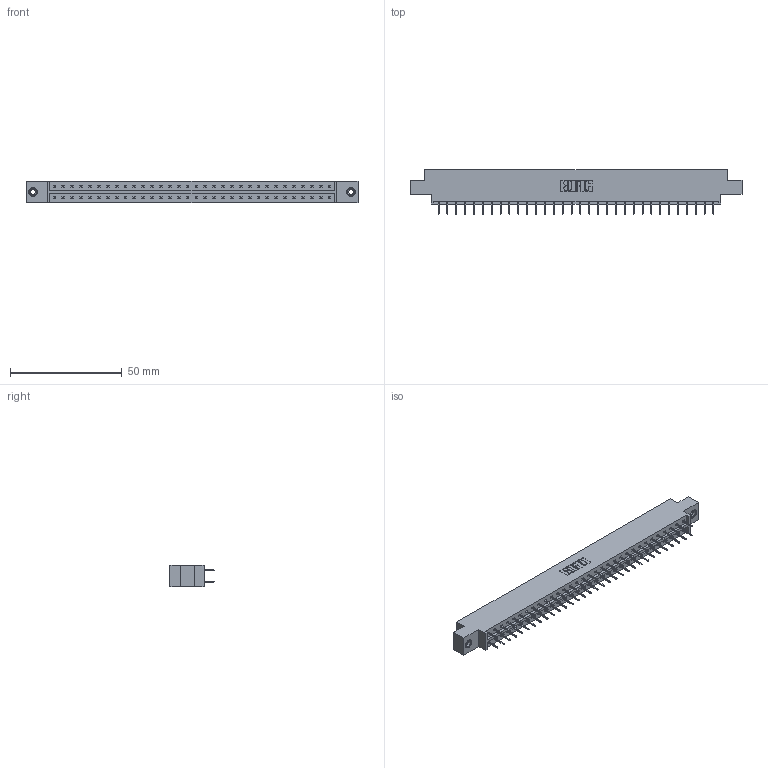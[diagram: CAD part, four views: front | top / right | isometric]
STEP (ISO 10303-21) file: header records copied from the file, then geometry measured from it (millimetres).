
FILE_DESCRIPTION (( 'STEP AP203' ), '1' );
FILE_NAME ('833-064-524-808.STEP', '2020-06-05T07:07:50', ( '' ), ( '' ), 'SwSTEP 2.0', 'SolidWorks 2020', '' );
FILE_SCHEMA (( 'CONFIG_CONTROL_DESIGN' ));
Length unit declared in the file: inch
Products named in the file (4): 833 Part_Offset - .156 Dia - TI; 833-064-524-808; 345-250-001_345-250-003-102; 345-292-001_345-293-124
Assembly tree (67 placements, depth 2):
  833-064-524-808
    833 Part_Offset - .156 Dia - TI
    345-292-001_345-293-124  x64
    345-250-001_345-250-003-102  x2
Bounding box: 148.34 x 19.69 x 9.4 mm (x, y, z)
Volume: 14719.6 mm3; surface area: 17246.6 mm2
Topology: 67 solids, 67 shells, 3762 faces, 10635 edges, 6826 vertices
Faces by surface type: plane 2794, cylinder 952, cone 12, torus 4
Entity records: 23272 total; most frequent: CARTESIAN_POINT 3853, ORIENTED_EDGE 3782, DIRECTION 3341, EDGE_CURVE 1891, VECTOR 1747, LINE 1747, VERTEX_POINT 1252, AXIS2_PLACEMENT_3D 797
